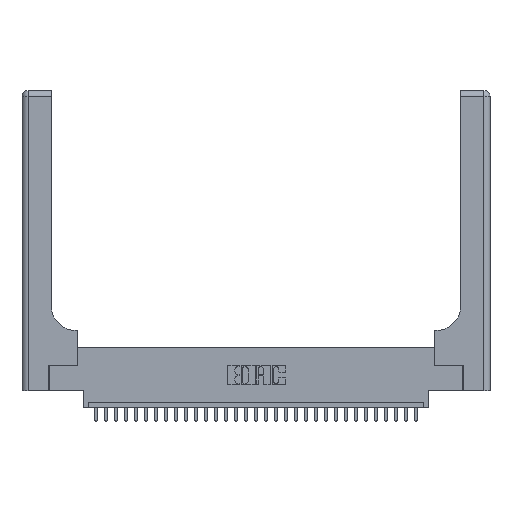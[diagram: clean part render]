
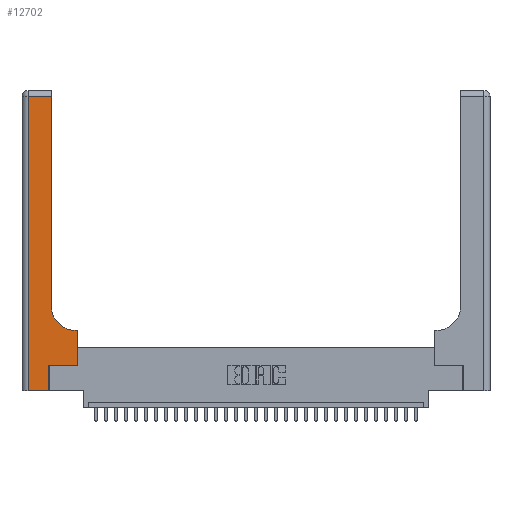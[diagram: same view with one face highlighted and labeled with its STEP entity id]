
A CAD part, top view. The second image highlights one B-rep face of the part: STEP entity #12702.
In plain terms, the highlighted planar face has unit normal (0, 0, 1).
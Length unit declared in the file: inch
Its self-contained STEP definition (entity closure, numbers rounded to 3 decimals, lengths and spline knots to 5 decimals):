
#577 = CARTESIAN_POINT ( 'NONE',  ( 0.5585, 0.25, 0.37 ) ) ;
#669 = CARTESIAN_POINT ( 'NONE',  ( 0.2915, 2.94, 0.37 ) ) ;
#1025 = ORIENTED_EDGE ( 'NONE', *, *, #10612, .T. ) ;
#1239 = LINE ( 'NONE', #11154, #11548 ) ;
#2067 = CARTESIAN_POINT ( 'NONE',  ( 0.06, 0., 0.37 ) ) ;
#2479 = DIRECTION ( 'NONE',  ( 0., 1., 0. ) ) ;
#2853 = VERTEX_POINT ( 'NONE', #24208 ) ;
#3091 = CARTESIAN_POINT ( 'NONE',  ( 0.269, 0., 0.37 ) ) ;
#3646 = ORIENTED_EDGE ( 'NONE', *, *, #27416, .T. ) ;
#4098 = CARTESIAN_POINT ( 'NONE',  ( 0.2915, 0.85, 0.37 ) ) ;
#5042 = EDGE_CURVE ( 'NONE', #2853, #10846, #7771, .T. ) ;
#5105 = CARTESIAN_POINT ( 'NONE',  ( 0.5585, 0.25, 0.37 ) ) ;
#5233 = FACE_OUTER_BOUND ( 'NONE', #10205, .T. ) ;
#5444 = VERTEX_POINT ( 'NONE', #25315 ) ;
#5803 = LINE ( 'NONE', #23632, #8479 ) ;
#6774 = VERTEX_POINT ( 'NONE', #25026 ) ;
#7349 = DIRECTION ( 'NONE',  ( 0., 1., 0. ) ) ;
#7435 = AXIS2_PLACEMENT_3D ( 'NONE', #27959, #13690, #30607 ) ;
#7620 = LINE ( 'NONE', #19549, #10256 ) ;
#7663 = AXIS2_PLACEMENT_3D ( 'NONE', #17446, #24587, #14878 ) ;
#7771 = LINE ( 'NONE', #20636, #12664 ) ;
#7963 = LINE ( 'NONE', #5105, #21944 ) ;
#8089 = DIRECTION ( 'NONE',  ( 0., 1., 0. ) ) ;
#8103 = EDGE_CURVE ( 'NONE', #6774, #2853, #18604, .T. ) ;
#8340 = EDGE_CURVE ( 'NONE', #28834, #14520, #7620, .T. ) ;
#8479 = VECTOR ( 'NONE', #23742, 39.37008 ) ;
#8577 = VERTEX_POINT ( 'NONE', #2067 ) ;
#9049 = EDGE_CURVE ( 'NONE', #15588, #9606, #1239, .T. ) ;
#9078 = ORIENTED_EDGE ( 'NONE', *, *, #11492, .T. ) ;
#9606 = VERTEX_POINT ( 'NONE', #21660 ) ;
#9704 = CARTESIAN_POINT ( 'NONE',  ( 0.5585, 0.6, 0.37 ) ) ;
#9732 = EDGE_CURVE ( 'NONE', #8577, #6774, #5803, .T. ) ;
#10205 = EDGE_LOOP ( 'NONE', ( #26582, #3646, #17706, #23756, #28076, #23383, #9078, #13407, #1025 ) ) ;
#10256 = VECTOR ( 'NONE', #2479, 39.37008 ) ;
#10612 = EDGE_CURVE ( 'NONE', #9606, #28834, #15201, .T. ) ;
#10846 = VERTEX_POINT ( 'NONE', #577 ) ;
#11154 = CARTESIAN_POINT ( 'NONE',  ( 0.2915, 0.6, 0.37 ) ) ;
#11492 = EDGE_CURVE ( 'NONE', #10846, #15588, #7963, .T. ) ;
#11548 = VECTOR ( 'NONE', #12617, 39.37008 ) ;
#12617 = DIRECTION ( 'NONE',  ( -1., 0., 0. ) ) ;
#12664 = VECTOR ( 'NONE', #25202, 39.37008 ) ;
#12702 = ADVANCED_FACE ( 'NONE', ( #5233 ), #27107, .F. ) ;
#13085 = CARTESIAN_POINT ( 'NONE',  ( 0.06, 3., 0.37 ) ) ;
#13361 = VECTOR ( 'NONE', #18427, 39.37008 ) ;
#13407 = ORIENTED_EDGE ( 'NONE', *, *, #9049, .T. ) ;
#13690 = DIRECTION ( 'NONE',  ( 0., 0., -1. ) ) ;
#14520 = VERTEX_POINT ( 'NONE', #669 ) ;
#14625 = VECTOR ( 'NONE', #30207, 39.37008 ) ;
#14878 = DIRECTION ( 'NONE',  ( -1., 0., 0. ) ) ;
#15201 = CIRCLE ( 'NONE', #7435, 0.25 ) ;
#15588 = VERTEX_POINT ( 'NONE', #9704 ) ;
#15854 = CARTESIAN_POINT ( 'NONE',  ( 0., 2.94, 0.37 ) ) ;
#16496 = EDGE_CURVE ( 'NONE', #5444, #8577, #20288, .T. ) ;
#17446 = CARTESIAN_POINT ( 'NONE',  ( 0., 3., 0.37 ) ) ;
#17706 = ORIENTED_EDGE ( 'NONE', *, *, #16496, .T. ) ;
#18427 = DIRECTION ( 'NONE',  ( -1., 0., 0. ) ) ;
#18604 = LINE ( 'NONE', #3091, #24244 ) ;
#19549 = CARTESIAN_POINT ( 'NONE',  ( 0.2915, 3., 0.37 ) ) ;
#20288 = LINE ( 'NONE', #13085, #14625 ) ;
#20636 = CARTESIAN_POINT ( 'NONE',  ( 0.269, 0.25, 0.37 ) ) ;
#21660 = CARTESIAN_POINT ( 'NONE',  ( 0.5415, 0.6, 0.37 ) ) ;
#21944 = VECTOR ( 'NONE', #7349, 39.37008 ) ;
#23383 = ORIENTED_EDGE ( 'NONE', *, *, #5042, .T. ) ;
#23632 = CARTESIAN_POINT ( 'NONE',  ( 0., 0., 0.37 ) ) ;
#23742 = DIRECTION ( 'NONE',  ( 1., 0., 0. ) ) ;
#23756 = ORIENTED_EDGE ( 'NONE', *, *, #9732, .T. ) ;
#24208 = CARTESIAN_POINT ( 'NONE',  ( 0.269, 0.25, 0.37 ) ) ;
#24244 = VECTOR ( 'NONE', #8089, 39.37008 ) ;
#24587 = DIRECTION ( 'NONE',  ( 0., 0., -1. ) ) ;
#24737 = LINE ( 'NONE', #15854, #13361 ) ;
#25026 = CARTESIAN_POINT ( 'NONE',  ( 0.269, 0., 0.37 ) ) ;
#25202 = DIRECTION ( 'NONE',  ( 1., 0., 0. ) ) ;
#25315 = CARTESIAN_POINT ( 'NONE',  ( 0.06, 2.94, 0.37 ) ) ;
#26582 = ORIENTED_EDGE ( 'NONE', *, *, #8340, .T. ) ;
#27107 = PLANE ( 'NONE',  #7663 ) ;
#27416 = EDGE_CURVE ( 'NONE', #14520, #5444, #24737, .T. ) ;
#27959 = CARTESIAN_POINT ( 'NONE',  ( 0.5415, 0.85, 0.37 ) ) ;
#28076 = ORIENTED_EDGE ( 'NONE', *, *, #8103, .T. ) ;
#28834 = VERTEX_POINT ( 'NONE', #4098 ) ;
#30207 = DIRECTION ( 'NONE',  ( 0., -1., 0. ) ) ;
#30607 = DIRECTION ( 'NONE',  ( 1., 0., 0. ) ) ;
